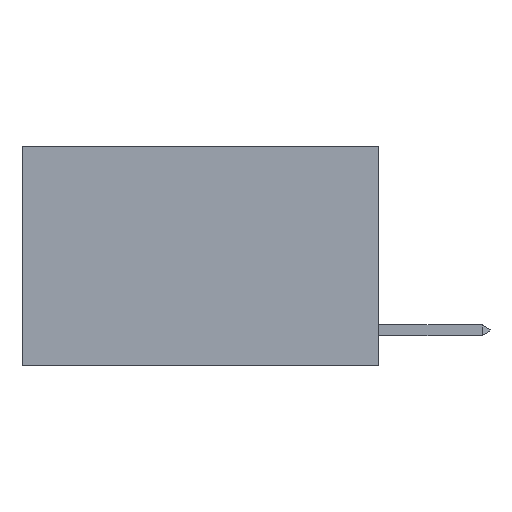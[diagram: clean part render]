
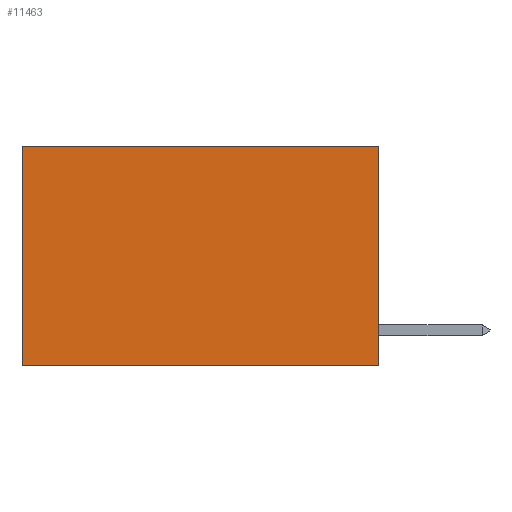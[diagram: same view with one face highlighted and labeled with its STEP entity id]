
A CAD part, left-side view. The second image highlights one B-rep face of the part: STEP entity #11463.
In plain terms, the highlighted planar face has unit normal (-1, 0, 0).
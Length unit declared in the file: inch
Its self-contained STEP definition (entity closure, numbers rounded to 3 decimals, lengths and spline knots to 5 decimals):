
#106 = LINE ( 'NONE', #8243, #14484 ) ;
#245 = CARTESIAN_POINT ( 'NONE',  ( 0.2625, 0.6, 0. ) ) ;
#1119 = EDGE_CURVE ( 'NONE', #20984, #17427, #17978, .T. ) ;
#1697 = DIRECTION ( 'NONE',  ( 1., 0., 0. ) ) ;
#2391 = DIRECTION ( 'NONE',  ( 0., 0., -1. ) ) ;
#2576 = ORIENTED_EDGE ( 'NONE', *, *, #7186, .T. ) ;
#3422 = DIRECTION ( 'NONE',  ( 0., 0., -1. ) ) ;
#3464 = VERTEX_POINT ( 'NONE', #20509 ) ;
#4252 = LINE ( 'NONE', #245, #15416 ) ;
#5550 = FACE_OUTER_BOUND ( 'NONE', #22430, .T. ) ;
#5794 = DIRECTION ( 'NONE',  ( 0., 1., 0. ) ) ;
#6593 = CARTESIAN_POINT ( 'NONE',  ( 0.2625, 0.6, 0. ) ) ;
#7033 = EDGE_CURVE ( 'NONE', #3464, #20984, #106, .T. ) ;
#7186 = EDGE_CURVE ( 'NONE', #19044, #17427, #4252, .T. ) ;
#7300 = CARTESIAN_POINT ( 'NONE',  ( 0.2625, 0., 0. ) ) ;
#7793 = CARTESIAN_POINT ( 'NONE',  ( 0.2625, 0., -0.37 ) ) ;
#8199 = ORIENTED_EDGE ( 'NONE', *, *, #1119, .F. ) ;
#8243 = CARTESIAN_POINT ( 'NONE',  ( 0.2625, 0., 0. ) ) ;
#8849 = EDGE_CURVE ( 'NONE', #3464, #19044, #25110, .T. ) ;
#11463 = ADVANCED_FACE ( 'NONE', ( #5550 ), #20008, .F. ) ;
#12229 = VECTOR ( 'NONE', #22703, 39.37008 ) ;
#14401 = ORIENTED_EDGE ( 'NONE', *, *, #7033, .F. ) ;
#14421 = DIRECTION ( 'NONE',  ( 0., 0., -1. ) ) ;
#14484 = VECTOR ( 'NONE', #14421, 39.37008 ) ;
#15416 = VECTOR ( 'NONE', #2391, 39.37008 ) ;
#17427 = VERTEX_POINT ( 'NONE', #17691 ) ;
#17428 = VECTOR ( 'NONE', #5794, 39.37008 ) ;
#17691 = CARTESIAN_POINT ( 'NONE',  ( 0.2625, 0.6, -0.37 ) ) ;
#17978 = LINE ( 'NONE', #7793, #17428 ) ;
#19044 = VERTEX_POINT ( 'NONE', #6593 ) ;
#19679 = CARTESIAN_POINT ( 'NONE',  ( 0.2625, 0., -0.37 ) ) ;
#20008 = PLANE ( 'NONE',  #24157 ) ;
#20509 = CARTESIAN_POINT ( 'NONE',  ( 0.2625, 0., 0. ) ) ;
#20984 = VERTEX_POINT ( 'NONE', #19679 ) ;
#21729 = CARTESIAN_POINT ( 'NONE',  ( 0.2625, 0., 0. ) ) ;
#22430 = EDGE_LOOP ( 'NONE', ( #2576, #8199, #14401, #23871 ) ) ;
#22703 = DIRECTION ( 'NONE',  ( 0., 1., 0. ) ) ;
#23871 = ORIENTED_EDGE ( 'NONE', *, *, #8849, .T. ) ;
#24157 = AXIS2_PLACEMENT_3D ( 'NONE', #21729, #1697, #3422 ) ;
#25110 = LINE ( 'NONE', #7300, #12229 ) ;
